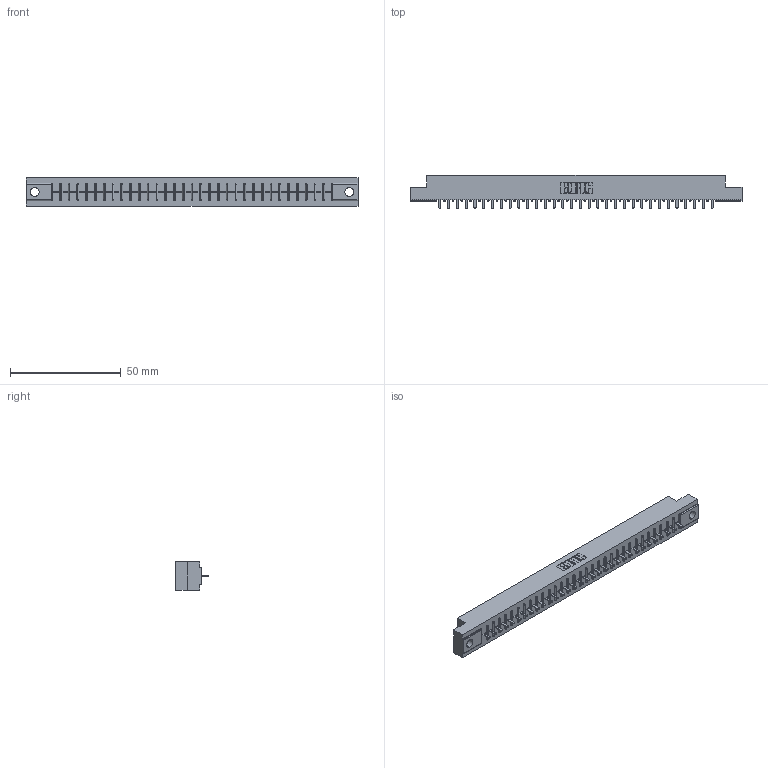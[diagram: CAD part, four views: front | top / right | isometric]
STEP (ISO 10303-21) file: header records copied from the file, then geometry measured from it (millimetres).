
FILE_DESCRIPTION (( 'STEP AP203' ), '1' );
FILE_NAME ('316-032-521-104.STEP', '2018-07-31T03:44:45', ( '' ), ( '' ), 'SwSTEP 2.0', 'SolidWorks 2016', '' );
FILE_SCHEMA (( 'CONFIG_CONTROL_DESIGN' ));
Length unit declared in the file: inch
Products named in the file (3): 306 Part_.156 Dia; 306-290-001_121; 316-032-521-104
Assembly tree (33 placements, depth 2):
  316-032-521-104
    306 Part_.156 Dia
    306-290-001_121  x32
Bounding box: 149.81 x 14.88 x 12.7 mm (x, y, z)
Volume: 16334.5 mm3; surface area: 16230.1 mm2
Topology: 33 solids, 33 shells, 2370 faces, 6656 edges, 4264 vertices
Faces by surface type: plane 1586, cylinder 656, sphere 128
Entity records: 31511 total; most frequent: CARTESIAN_POINT 5293, ORIENTED_EDGE 5244, DIRECTION 5212, EDGE_CURVE 2622, LINE 2054, VECTOR 2054, VERTEX_POINT 1660, AXIS2_PLACEMENT_3D 1579
